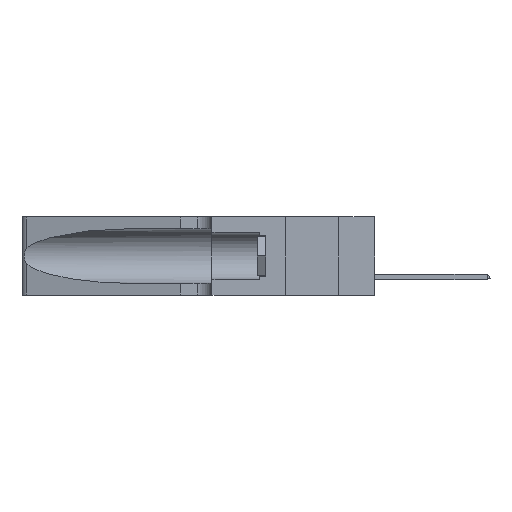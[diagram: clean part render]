
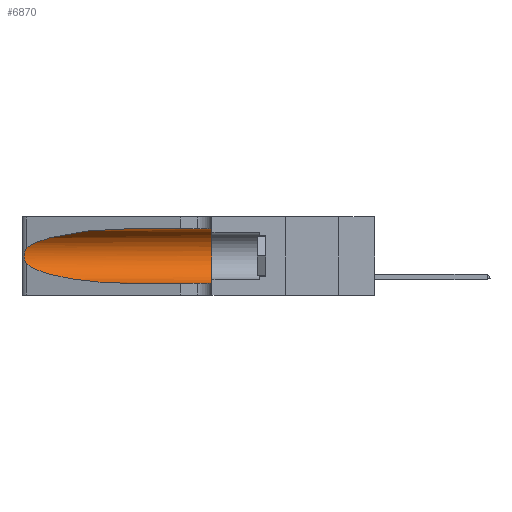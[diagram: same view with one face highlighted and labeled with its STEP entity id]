
A CAD part, left-side view. The second image highlights one B-rep face of the part: STEP entity #6870.
In plain terms, the highlighted cylindrical face has radius 3.308 mm (diameter 6.617 mm), a partial arc.
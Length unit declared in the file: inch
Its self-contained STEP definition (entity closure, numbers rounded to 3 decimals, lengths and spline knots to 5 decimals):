
#385 = CARTESIAN_POINT ( 'NONE',  ( 0.25487, 1.22718, 0.22369 ) ) ;
#889 = EDGE_CURVE ( 'NONE', #1461, #29471, #17481, .T. ) ;
#1121 =( BOUNDED_CURVE ( )  B_SPLINE_CURVE ( 3, ( #23004, #29837, #39992, #19455 ),
 .UNSPECIFIED., .F., .T. ) 
 B_SPLINE_CURVE_WITH_KNOTS ( ( 4, 4 ),
 ( 3.44316, 4.71239 ),
 .UNSPECIFIED. ) 
 CURVE ( )  GEOMETRIC_REPRESENTATION_ITEM ( )  RATIONAL_B_SPLINE_CURVE ( ( 1., 0.87, 0.87, 1. ) ) 
 REPRESENTATION_ITEM ( '' )  );
#1461 = VERTEX_POINT ( 'NONE', #35600 ) ;
#2930 = DIRECTION ( 'NONE',  ( 0., 0., 1. ) ) ;
#3069 = EDGE_CURVE ( 'NONE', #1461, #7623, #15176, .T. ) ;
#4914 = CARTESIAN_POINT ( 'NONE',  ( 0.25639, 1.23184, 0.21858 ) ) ;
#5074 = CARTESIAN_POINT ( 'NONE',  ( 0.25555, 1.22993, 0.14849 ) ) ;
#6388 = ORIENTED_EDGE ( 'NONE', *, *, #23235, .T. ) ;
#6842 = ORIENTED_EDGE ( 'NONE', *, *, #23357, .T. ) ;
#6870 = ADVANCED_FACE ( 'NONE', ( #24920 ), #18543, .F. ) ;
#7623 = VERTEX_POINT ( 'NONE', #32351 ) ;
#7744 = CARTESIAN_POINT ( 'NONE',  ( 0.25555, 1.22994, 0.2215 ) ) ;
#7778 = ORIENTED_EDGE ( 'NONE', *, *, #3069, .F. ) ;
#7847 = CARTESIAN_POINT ( 'NONE',  ( 0.1305, 1.61858, 0.31525 ) ) ;
#8985 = CARTESIAN_POINT ( 'NONE',  ( 0.25787, 1.23484, 0.2124 ) ) ;
#9370 = EDGE_CURVE ( 'NONE', #43104, #16527, #1121, .T. ) ;
#9674 = DIRECTION ( 'NONE',  ( 0., 0., -1. ) ) ;
#10972 = CARTESIAN_POINT ( 'NONE',  ( 0.1305, 0.72297, 0.31525 ) ) ;
#11948 = CARTESIAN_POINT ( 'NONE',  ( 0.25487, 1.22718, 0.14631 ) ) ;
#12246 = CARTESIAN_POINT ( 'NONE',  ( 0.26075, 1.23896, 0.19203 ) ) ;
#12785 = ORIENTED_EDGE ( 'NONE', *, *, #889, .T. ) ;
#13039 = DIRECTION ( 'NONE',  ( 0., -1., 0. ) ) ;
#13181 = CARTESIAN_POINT ( 'NONE',  ( 0.25487, 1.22718, 0.14631 ) ) ;
#13617 = VECTOR ( 'NONE', #23286, 39.37008 ) ;
#15176 = LINE ( 'NONE', #7847, #13617 ) ;
#15619 = CARTESIAN_POINT ( 'NONE',  ( 0.25639, 1.23186, 0.15144 ) ) ;
#15986 = CARTESIAN_POINT ( 'NONE',  ( 0.1305, 0.72297, 0.05475 ) ) ;
#16271 = CIRCLE ( 'NONE', #36411, 0.13025 ) ;
#16527 = VERTEX_POINT ( 'NONE', #15986 ) ;
#17481 =( BOUNDED_CURVE ( )  B_SPLINE_CURVE ( 3, ( #10972, #21181, #20758, #385 ),
 .UNSPECIFIED., .F., .F. ) 
 B_SPLINE_CURVE_WITH_KNOTS ( ( 4, 4 ),
 ( 1.5708, 2.84003 ),
 .UNSPECIFIED. ) 
 CURVE ( )  GEOMETRIC_REPRESENTATION_ITEM ( )  RATIONAL_B_SPLINE_CURVE ( ( 1., 0.87, 0.87, 1. ) ) 
 REPRESENTATION_ITEM ( '' )  );
#17669 = CARTESIAN_POINT ( 'NONE',  ( 0.25487, 1.22718, 0.22369 ) ) ;
#18009 = CARTESIAN_POINT ( 'NONE',  ( 0.25487, 1.22718, 0.22369 ) ) ;
#18543 = CYLINDRICAL_SURFACE ( 'NONE', #37793, 0.13025 ) ;
#18636 = ORIENTED_EDGE ( 'NONE', *, *, #9370, .T. ) ;
#19455 = CARTESIAN_POINT ( 'NONE',  ( 0.1305, 0.72297, 0.05475 ) ) ;
#20758 = CARTESIAN_POINT ( 'NONE',  ( 0.2373, 1.15595, 0.28018 ) ) ;
#21181 = CARTESIAN_POINT ( 'NONE',  ( 0.18966, 0.96281, 0.31525 ) ) ;
#23004 = CARTESIAN_POINT ( 'NONE',  ( 0.25487, 1.22718, 0.14631 ) ) ;
#23235 = EDGE_CURVE ( 'NONE', #16527, #32633, #33273, .T. ) ;
#23286 = DIRECTION ( 'NONE',  ( 0., -1., 0. ) ) ;
#23357 = EDGE_CURVE ( 'NONE', #29471, #43104, #41026, .T. ) ;
#24920 = FACE_OUTER_BOUND ( 'NONE', #29632, .T. ) ;
#26720 = DIRECTION ( 'NONE',  ( 0., 1., 0. ) ) ;
#27367 = EDGE_CURVE ( 'NONE', #7623, #32633, #16271, .T. ) ;
#29471 = VERTEX_POINT ( 'NONE', #18009 ) ;
#29632 = EDGE_LOOP ( 'NONE', ( #12785, #6842, #18636, #6388, #31953, #7778 ) ) ;
#29837 = CARTESIAN_POINT ( 'NONE',  ( 0.2373, 1.15595, 0.08982 ) ) ;
#30319 = CARTESIAN_POINT ( 'NONE',  ( 0.1305, 1.61858, 0.05475 ) ) ;
#31953 = ORIENTED_EDGE ( 'NONE', *, *, #27367, .F. ) ;
#32200 = CARTESIAN_POINT ( 'NONE',  ( 0.25854, 1.2359, 0.20912 ) ) ;
#32351 = CARTESIAN_POINT ( 'NONE',  ( 0.1305, 0.35, 0.31525 ) ) ;
#32358 = CARTESIAN_POINT ( 'NONE',  ( 0.25856, 1.23593, 0.16098 ) ) ;
#32633 = VERTEX_POINT ( 'NONE', #34053 ) ;
#33273 = LINE ( 'NONE', #30319, #42717 ) ;
#33509 = CARTESIAN_POINT ( 'NONE',  ( 0.1305, 1.61858, 0.185 ) ) ;
#33882 = CARTESIAN_POINT ( 'NONE',  ( 0.1305, 0.35, 0.185 ) ) ;
#34053 = CARTESIAN_POINT ( 'NONE',  ( 0.1305, 0.35, 0.05475 ) ) ;
#35243 = CARTESIAN_POINT ( 'NONE',  ( 0.26018, 1.23835, 0.19895 ) ) ;
#35600 = CARTESIAN_POINT ( 'NONE',  ( 0.1305, 0.72297, 0.31525 ) ) ;
#36411 = AXIS2_PLACEMENT_3D ( 'NONE', #33882, #26720, #2930 ) ;
#37793 = AXIS2_PLACEMENT_3D ( 'NONE', #33509, #40291, #9674 ) ;
#38803 = CARTESIAN_POINT ( 'NONE',  ( 0.26075, 1.23896, 0.178 ) ) ;
#39992 = CARTESIAN_POINT ( 'NONE',  ( 0.18966, 0.96281, 0.05475 ) ) ;
#40291 = DIRECTION ( 'NONE',  ( 0., -1., 0. ) ) ;
#41026 = B_SPLINE_CURVE_WITH_KNOTS ( 'NONE', 3,
 ( #17669, #7744, #4914, #8985, #32200, #35243, #12246, #38803, #42499, #32358, #42199, #15619, #5074, #11948 ),
 .UNSPECIFIED., .F., .F.,
 ( 4, 2, 2, 2, 2, 2, 4 ),
 ( 0., 0.00027, 0.00053, 0.00107, 0.0016, 0.00187, 0.00214 ),
 .UNSPECIFIED. ) ;
#42199 = CARTESIAN_POINT ( 'NONE',  ( 0.25789, 1.23486, 0.15765 ) ) ;
#42499 = CARTESIAN_POINT ( 'NONE',  ( 0.26017, 1.23833, 0.17102 ) ) ;
#42717 = VECTOR ( 'NONE', #13039, 39.37008 ) ;
#43104 = VERTEX_POINT ( 'NONE', #13181 ) ;
